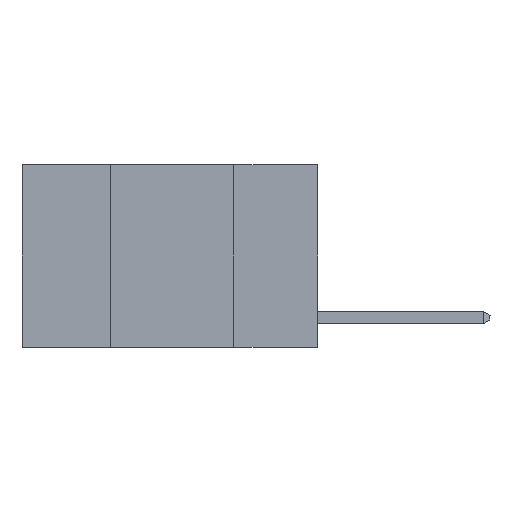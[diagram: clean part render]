
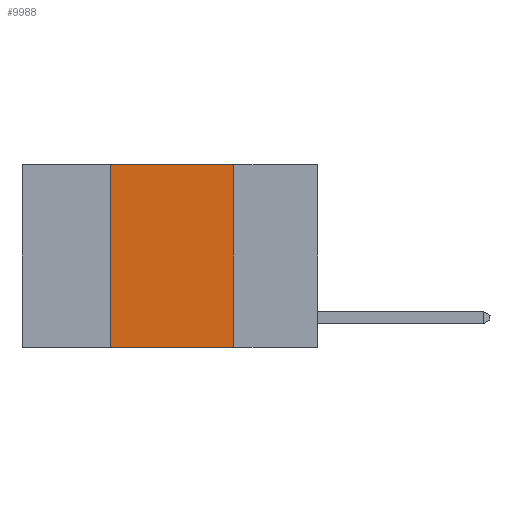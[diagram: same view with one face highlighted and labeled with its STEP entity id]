
A CAD part, left-side view. The second image highlights one B-rep face of the part: STEP entity #9988.
In plain terms, the highlighted planar face has unit normal (-1, 0, 0).
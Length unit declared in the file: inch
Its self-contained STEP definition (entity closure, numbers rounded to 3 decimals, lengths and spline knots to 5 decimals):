
#223 = VECTOR ( 'NONE', #17818, 39.37008 ) ;
#266 = LINE ( 'NONE', #5365, #12106 ) ;
#1541 = CARTESIAN_POINT ( 'NONE',  ( 0., 0.17, -0.37 ) ) ;
#1599 = EDGE_CURVE ( 'NONE', #9623, #2362, #14877, .T. ) ;
#2294 = DIRECTION ( 'NONE',  ( 0., -1., 0. ) ) ;
#2326 = ORIENTED_EDGE ( 'NONE', *, *, #13661, .F. ) ;
#2362 = VERTEX_POINT ( 'NONE', #8810 ) ;
#2864 = CARTESIAN_POINT ( 'NONE',  ( 0., 0.6, 0. ) ) ;
#4122 = LINE ( 'NONE', #14836, #223 ) ;
#4253 = CARTESIAN_POINT ( 'NONE',  ( 0., 0.42, -0.37 ) ) ;
#5321 = AXIS2_PLACEMENT_3D ( 'NONE', #2864, #12044, #13919 ) ;
#5365 = CARTESIAN_POINT ( 'NONE',  ( 0., 0.17, 0. ) ) ;
#7413 = DIRECTION ( 'NONE',  ( 0., 0., 1. ) ) ;
#8810 = CARTESIAN_POINT ( 'NONE',  ( 0., 0.17, 0. ) ) ;
#8814 = EDGE_LOOP ( 'NONE', ( #15214, #10121, #2326, #14070 ) ) ;
#9207 = VERTEX_POINT ( 'NONE', #4253 ) ;
#9429 = VERTEX_POINT ( 'NONE', #1541 ) ;
#9623 = VERTEX_POINT ( 'NONE', #18535 ) ;
#9988 = ADVANCED_FACE ( 'NONE', ( #16066 ), #14939, .F. ) ;
#10121 = ORIENTED_EDGE ( 'NONE', *, *, #1599, .F. ) ;
#11403 = CARTESIAN_POINT ( 'NONE',  ( 0., 0.6, 0. ) ) ;
#11556 = LINE ( 'NONE', #14800, #14696 ) ;
#12044 = DIRECTION ( 'NONE',  ( 1., 0., 0. ) ) ;
#12106 = VECTOR ( 'NONE', #14467, 39.37008 ) ;
#13661 = EDGE_CURVE ( 'NONE', #9207, #9623, #11556, .T. ) ;
#13919 = DIRECTION ( 'NONE',  ( 0., 0., -1. ) ) ;
#14070 = ORIENTED_EDGE ( 'NONE', *, *, #19814, .T. ) ;
#14467 = DIRECTION ( 'NONE',  ( 0., 0., -1. ) ) ;
#14696 = VECTOR ( 'NONE', #7413, 39.37008 ) ;
#14800 = CARTESIAN_POINT ( 'NONE',  ( 0., 0.42, 0. ) ) ;
#14836 = CARTESIAN_POINT ( 'NONE',  ( 0., 0.6, -0.37 ) ) ;
#14877 = LINE ( 'NONE', #11403, #17260 ) ;
#14939 = PLANE ( 'NONE',  #5321 ) ;
#15214 = ORIENTED_EDGE ( 'NONE', *, *, #18944, .F. ) ;
#16066 = FACE_OUTER_BOUND ( 'NONE', #8814, .T. ) ;
#17260 = VECTOR ( 'NONE', #2294, 39.37008 ) ;
#17818 = DIRECTION ( 'NONE',  ( 0., -1., 0. ) ) ;
#18535 = CARTESIAN_POINT ( 'NONE',  ( 0., 0.42, 0. ) ) ;
#18944 = EDGE_CURVE ( 'NONE', #2362, #9429, #266, .T. ) ;
#19814 = EDGE_CURVE ( 'NONE', #9207, #9429, #4122, .T. ) ;
